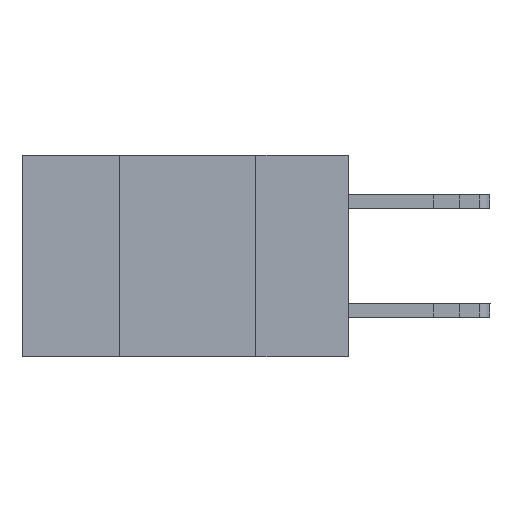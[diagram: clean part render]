
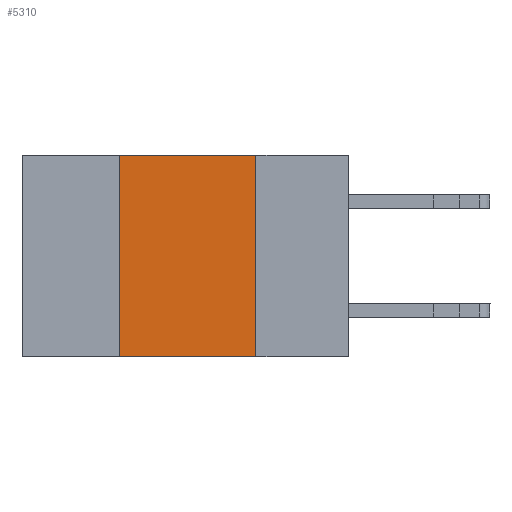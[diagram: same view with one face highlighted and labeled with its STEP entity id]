
A CAD part, left-side view. The second image highlights one B-rep face of the part: STEP entity #5310.
In plain terms, the highlighted planar face has unit normal (-1, 0, 0).
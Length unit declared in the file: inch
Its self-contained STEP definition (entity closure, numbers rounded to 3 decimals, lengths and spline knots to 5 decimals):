
#436 = LINE ( 'NONE', #4868, #9985 ) ;
#480 = DIRECTION ( 'NONE',  ( 0., -1., 0. ) ) ;
#771 = ORIENTED_EDGE ( 'NONE', *, *, #9634, .F. ) ;
#779 = ORIENTED_EDGE ( 'NONE', *, *, #5998, .F. ) ;
#825 = ORIENTED_EDGE ( 'NONE', *, *, #5392, .F. ) ;
#837 = ORIENTED_EDGE ( 'NONE', *, *, #4115, .T. ) ;
#1419 = DIRECTION ( 'NONE',  ( 1., 0., 0. ) ) ;
#2481 = DIRECTION ( 'NONE',  ( 0., 0., 1. ) ) ;
#3219 = LINE ( 'NONE', #6485, #7836 ) ;
#3715 = CARTESIAN_POINT ( 'NONE',  ( 0., 0.17, 0. ) ) ;
#3929 = VERTEX_POINT ( 'NONE', #6698 ) ;
#4022 = VECTOR ( 'NONE', #480, 39.37008 ) ;
#4115 = EDGE_CURVE ( 'NONE', #3929, #5141, #436, .T. ) ;
#4212 = CARTESIAN_POINT ( 'NONE',  ( 0., 0.6, 0. ) ) ;
#4741 = DIRECTION ( 'NONE',  ( 0., -1., 0. ) ) ;
#4868 = CARTESIAN_POINT ( 'NONE',  ( 0., 0.6, -0.37 ) ) ;
#4923 = CARTESIAN_POINT ( 'NONE',  ( 0., 0.17, -0.37 ) ) ;
#5141 = VERTEX_POINT ( 'NONE', #4923 ) ;
#5310 = ADVANCED_FACE ( 'NONE', ( #10840 ), #6976, .F. ) ;
#5392 = EDGE_CURVE ( 'NONE', #3929, #9010, #9754, .T. ) ;
#5998 = EDGE_CURVE ( 'NONE', #9010, #8292, #10958, .T. ) ;
#6485 = CARTESIAN_POINT ( 'NONE',  ( 0., 0.17, -0.37 ) ) ;
#6698 = CARTESIAN_POINT ( 'NONE',  ( 0., 0.42, -0.37 ) ) ;
#6947 = AXIS2_PLACEMENT_3D ( 'NONE', #4212, #1419, #7914 ) ;
#6976 = PLANE ( 'NONE',  #6947 ) ;
#7000 = CARTESIAN_POINT ( 'NONE',  ( 0., 0.6, 0. ) ) ;
#7386 = DIRECTION ( 'NONE',  ( 0., 0., -1. ) ) ;
#7639 = VECTOR ( 'NONE', #2481, 39.37008 ) ;
#7836 = VECTOR ( 'NONE', #7386, 39.37008 ) ;
#7914 = DIRECTION ( 'NONE',  ( 0., 0., -1. ) ) ;
#8036 = CARTESIAN_POINT ( 'NONE',  ( 0., 0.42, -0.37 ) ) ;
#8292 = VERTEX_POINT ( 'NONE', #3715 ) ;
#8393 = CARTESIAN_POINT ( 'NONE',  ( 0., 0.42, 0. ) ) ;
#9010 = VERTEX_POINT ( 'NONE', #8393 ) ;
#9634 = EDGE_CURVE ( 'NONE', #8292, #5141, #3219, .T. ) ;
#9754 = LINE ( 'NONE', #8036, #7639 ) ;
#9985 = VECTOR ( 'NONE', #4741, 39.37008 ) ;
#10526 = EDGE_LOOP ( 'NONE', ( #771, #779, #825, #837 ) ) ;
#10840 = FACE_OUTER_BOUND ( 'NONE', #10526, .T. ) ;
#10958 = LINE ( 'NONE', #7000, #4022 ) ;
